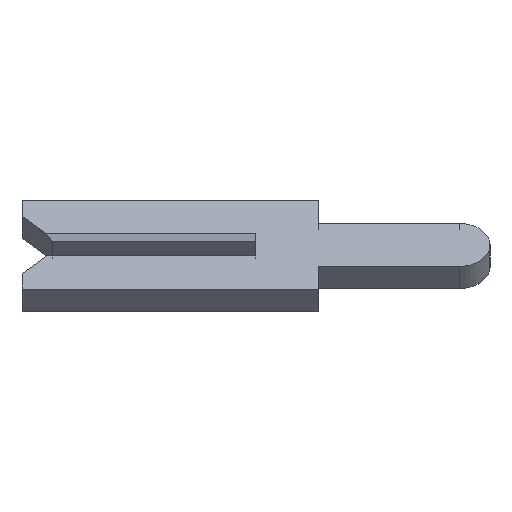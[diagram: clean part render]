
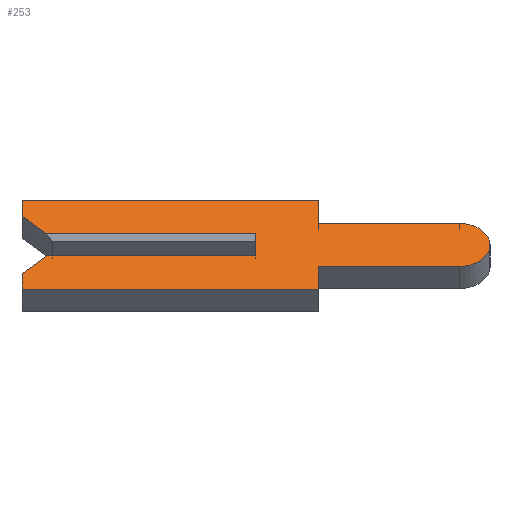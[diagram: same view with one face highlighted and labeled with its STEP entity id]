
A CAD part, left-side view. The second image highlights one B-rep face of the part: STEP entity #253.
In plain terms, the highlighted face is planar.
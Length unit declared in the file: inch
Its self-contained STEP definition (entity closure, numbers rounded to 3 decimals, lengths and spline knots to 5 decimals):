
#5 = LINE ( 'NONE', #616, #448 ) ;
#15 = CARTESIAN_POINT ( 'NONE',  ( -0.01, -0.04, 0.04 ) ) ;
#22 = EDGE_CURVE ( 'NONE', #864, #773, #299, .T. ) ;
#41 = CARTESIAN_POINT ( 'NONE',  ( -0.01, -0.04, -0.0195 ) ) ;
#44 = VERTEX_POINT ( 'NONE', #755 ) ;
#48 = CARTESIAN_POINT ( 'NONE',  ( -0.01, 0.134, 0.01 ) ) ;
#54 = ORIENTED_EDGE ( 'NONE', *, *, #128, .F. ) ;
#59 = DIRECTION ( 'NONE',  ( 0., 1., 0. ) ) ;
#61 = EDGE_LOOP ( 'NONE', ( #1139, #620, #818, #245, #196, #261, #845, #672, #74, #596, #583, #351, #213, #54 ) ) ;
#69 = LINE ( 'NONE', #1127, #207 ) ;
#70 = VECTOR ( 'NONE', #1041, 39.37008 ) ;
#71 = CARTESIAN_POINT ( 'NONE',  ( -0.01, 0.15, -0.04 ) ) ;
#74 = ORIENTED_EDGE ( 'NONE', *, *, #567, .F. ) ;
#126 = VERTEX_POINT ( 'NONE', #501 ) ;
#128 = EDGE_CURVE ( 'NONE', #890, #352, #69, .T. ) ;
#134 = LINE ( 'NONE', #758, #673 ) ;
#148 = FACE_OUTER_BOUND ( 'NONE', #61, .T. ) ;
#151 = DIRECTION ( 'NONE',  ( 0., 1., 0. ) ) ;
#175 = DIRECTION ( 'NONE',  ( 0., -0.707, 0.707 ) ) ;
#187 = EDGE_CURVE ( 'NONE', #890, #435, #331, .T. ) ;
#193 = LINE ( 'NONE', #333, #644 ) ;
#196 = ORIENTED_EDGE ( 'NONE', *, *, #1098, .F. ) ;
#207 = VECTOR ( 'NONE', #217, 39.37008 ) ;
#213 = ORIENTED_EDGE ( 'NONE', *, *, #485, .F. ) ;
#217 = DIRECTION ( 'NONE',  ( 0., 0.707, 0.707 ) ) ;
#222 = CARTESIAN_POINT ( 'NONE',  ( -0.01, -0.1305, -0.0195 ) ) ;
#227 = CARTESIAN_POINT ( 'NONE',  ( -0.01, -0.04, -0.04 ) ) ;
#245 = ORIENTED_EDGE ( 'NONE', *, *, #384, .F. ) ;
#253 = ADVANCED_FACE ( 'NONE', ( #148 ), #511, .F. ) ;
#261 = ORIENTED_EDGE ( 'NONE', *, *, #1112, .F. ) ;
#275 = VECTOR ( 'NONE', #741, 39.37008 ) ;
#276 = DIRECTION ( 'NONE',  ( 0., 0., -1. ) ) ;
#295 = CARTESIAN_POINT ( 'NONE',  ( -0.01, 0., -0.01 ) ) ;
#299 = LINE ( 'NONE', #592, #921 ) ;
#301 = CIRCLE ( 'NONE', #717, 0.0195 ) ;
#302 = CARTESIAN_POINT ( 'NONE',  ( -0.01, 0., 0.0065 ) ) ;
#319 = VECTOR ( 'NONE', #1103, 39.37008 ) ;
#321 = CARTESIAN_POINT ( 'NONE',  ( -0.01, -0.04, -0.04 ) ) ;
#331 = LINE ( 'NONE', #1138, #392 ) ;
#333 = CARTESIAN_POINT ( 'NONE',  ( -0.01, 0.15, -0.026 ) ) ;
#351 = ORIENTED_EDGE ( 'NONE', *, *, #1072, .F. ) ;
#352 = VERTEX_POINT ( 'NONE', #1053 ) ;
#367 = DIRECTION ( 'NONE',  ( 0., 0., -1. ) ) ;
#369 = DIRECTION ( 'NONE',  ( 0., 0., 1. ) ) ;
#384 = EDGE_CURVE ( 'NONE', #742, #126, #5, .T. ) ;
#392 = VECTOR ( 'NONE', #1048, 39.37008 ) ;
#396 = CARTESIAN_POINT ( 'NONE',  ( -0.01, -0.04, 0.04 ) ) ;
#410 = DIRECTION ( 'NONE',  ( 0., -1., 0. ) ) ;
#429 = DIRECTION ( 'NONE',  ( 1., 0., 0. ) ) ;
#431 = LINE ( 'NONE', #71, #877 ) ;
#435 = VERTEX_POINT ( 'NONE', #686 ) ;
#440 = EDGE_CURVE ( 'NONE', #688, #44, #604, .T. ) ;
#447 = VECTOR ( 'NONE', #367, 39.37008 ) ;
#448 = VECTOR ( 'NONE', #175, 39.37008 ) ;
#459 = CARTESIAN_POINT ( 'NONE',  ( -0.01, -0.1305, -0.01 ) ) ;
#485 = EDGE_CURVE ( 'NONE', #352, #707, #878, .T. ) ;
#488 = LINE ( 'NONE', #459, #1026 ) ;
#501 = CARTESIAN_POINT ( 'NONE',  ( -0.01, 0.134, -0.01 ) ) ;
#511 = PLANE ( 'NONE',  #700 ) ;
#530 = EDGE_CURVE ( 'NONE', #126, #637, #488, .T. ) ;
#562 = CARTESIAN_POINT ( 'NONE',  ( -0.01, -0.1305, 0.0195 ) ) ;
#567 = EDGE_CURVE ( 'NONE', #585, #864, #301, .T. ) ;
#573 = CARTESIAN_POINT ( 'NONE',  ( -0.01, 0.15, -0.026 ) ) ;
#583 = ORIENTED_EDGE ( 'NONE', *, *, #440, .F. ) ;
#585 = VERTEX_POINT ( 'NONE', #562 ) ;
#592 = CARTESIAN_POINT ( 'NONE',  ( -0.01, -0.04, -0.0195 ) ) ;
#595 = DIRECTION ( 'NONE',  ( 0., 0., -1. ) ) ;
#596 = ORIENTED_EDGE ( 'NONE', *, *, #617, .F. ) ;
#604 = LINE ( 'NONE', #15, #447 ) ;
#616 = CARTESIAN_POINT ( 'NONE',  ( -0.01, 0.1305, -0.0065 ) ) ;
#617 = EDGE_CURVE ( 'NONE', #44, #585, #646, .T. ) ;
#619 = DIRECTION ( 'NONE',  ( 0., 0., 1. ) ) ;
#620 = ORIENTED_EDGE ( 'NONE', *, *, #647, .F. ) ;
#637 = VERTEX_POINT ( 'NONE', #295 ) ;
#644 = VECTOR ( 'NONE', #619, 39.37008 ) ;
#646 = LINE ( 'NONE', #834, #275 ) ;
#647 = EDGE_CURVE ( 'NONE', #637, #435, #936, .T. ) ;
#667 = CARTESIAN_POINT ( 'NONE',  ( -0.01, 0.15, 0.04 ) ) ;
#672 = ORIENTED_EDGE ( 'NONE', *, *, #22, .F. ) ;
#673 = VECTOR ( 'NONE', #410, 39.37008 ) ;
#686 = CARTESIAN_POINT ( 'NONE',  ( -0.01, 0., 0.01 ) ) ;
#688 = VERTEX_POINT ( 'NONE', #396 ) ;
#700 = AXIS2_PLACEMENT_3D ( 'NONE', #780, #429, #595 ) ;
#707 = VERTEX_POINT ( 'NONE', #667 ) ;
#717 = AXIS2_PLACEMENT_3D ( 'NONE', #1086, #1094, #276 ) ;
#726 = VECTOR ( 'NONE', #369, 39.37008 ) ;
#741 = DIRECTION ( 'NONE',  ( 0., -1., 0. ) ) ;
#742 = VERTEX_POINT ( 'NONE', #573 ) ;
#755 = CARTESIAN_POINT ( 'NONE',  ( -0.01, -0.04, 0.0195 ) ) ;
#758 = CARTESIAN_POINT ( 'NONE',  ( -0.01, 0.15, 0.04 ) ) ;
#773 = VERTEX_POINT ( 'NONE', #41 ) ;
#780 = CARTESIAN_POINT ( 'NONE',  ( -0.01, -0.1305, 0. ) ) ;
#808 = CARTESIAN_POINT ( 'NONE',  ( -0.01, 0.15, 0.026 ) ) ;
#818 = ORIENTED_EDGE ( 'NONE', *, *, #530, .F. ) ;
#834 = CARTESIAN_POINT ( 'NONE',  ( -0.01, -0.04, 0.0195 ) ) ;
#845 = ORIENTED_EDGE ( 'NONE', *, *, #1134, .F. ) ;
#855 = CARTESIAN_POINT ( 'NONE',  ( -0.01, 0.15, -0.04 ) ) ;
#864 = VERTEX_POINT ( 'NONE', #222 ) ;
#877 = VECTOR ( 'NONE', #151, 39.37008 ) ;
#878 = LINE ( 'NONE', #808, #726 ) ;
#890 = VERTEX_POINT ( 'NONE', #48 ) ;
#921 = VECTOR ( 'NONE', #59, 39.37008 ) ;
#936 = LINE ( 'NONE', #302, #319 ) ;
#956 = VERTEX_POINT ( 'NONE', #855 ) ;
#1026 = VECTOR ( 'NONE', #1087, 39.37008 ) ;
#1028 = VERTEX_POINT ( 'NONE', #321 ) ;
#1041 = DIRECTION ( 'NONE',  ( 0., 0., -1. ) ) ;
#1048 = DIRECTION ( 'NONE',  ( 0., -1., 0. ) ) ;
#1053 = CARTESIAN_POINT ( 'NONE',  ( -0.01, 0.15, 0.026 ) ) ;
#1062 = LINE ( 'NONE', #227, #70 ) ;
#1072 = EDGE_CURVE ( 'NONE', #707, #688, #134, .T. ) ;
#1086 = CARTESIAN_POINT ( 'NONE',  ( -0.01, -0.1305, 0. ) ) ;
#1087 = DIRECTION ( 'NONE',  ( 0., -1., 0. ) ) ;
#1094 = DIRECTION ( 'NONE',  ( 1., 0., 0. ) ) ;
#1098 = EDGE_CURVE ( 'NONE', #956, #742, #193, .T. ) ;
#1103 = DIRECTION ( 'NONE',  ( 0., 0., 1. ) ) ;
#1112 = EDGE_CURVE ( 'NONE', #1028, #956, #431, .T. ) ;
#1127 = CARTESIAN_POINT ( 'NONE',  ( -0.01, 0.1305, 0.0065 ) ) ;
#1134 = EDGE_CURVE ( 'NONE', #773, #1028, #1062, .T. ) ;
#1138 = CARTESIAN_POINT ( 'NONE',  ( -0.01, 0.15, 0.01 ) ) ;
#1139 = ORIENTED_EDGE ( 'NONE', *, *, #187, .T. ) ;
